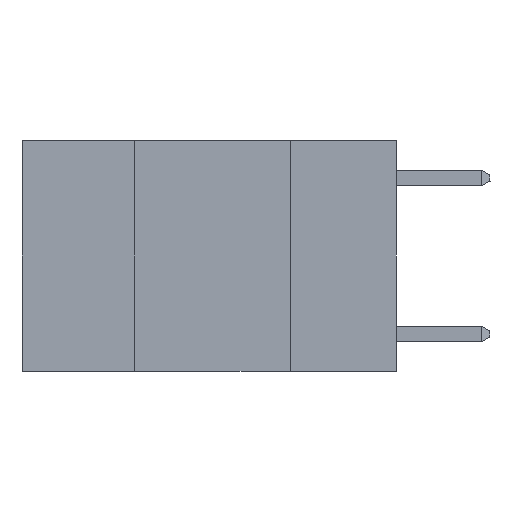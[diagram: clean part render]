
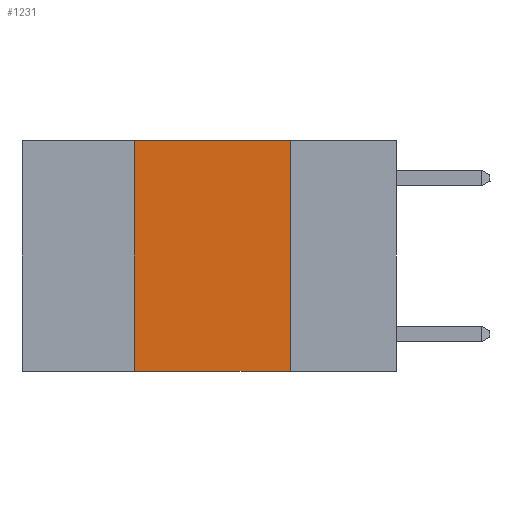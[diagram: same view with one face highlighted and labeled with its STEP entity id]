
A CAD part, left-side view. The second image highlights one B-rep face of the part: STEP entity #1231.
In plain terms, the highlighted planar face has unit normal (-1, 0, 0).
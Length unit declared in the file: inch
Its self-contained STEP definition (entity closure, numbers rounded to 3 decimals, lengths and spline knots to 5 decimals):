
#757 = VECTOR ( 'NONE', #13099, 39.37008 ) ;
#1231 = ADVANCED_FACE ( 'NONE', ( #10437 ), #6418, .F. ) ;
#1411 = CARTESIAN_POINT ( 'NONE',  ( 0., 0.42, -0.37 ) ) ;
#2213 = EDGE_LOOP ( 'NONE', ( #12936, #3602, #9291, #8580 ) ) ;
#2534 = CARTESIAN_POINT ( 'NONE',  ( 0., 0.17, 0. ) ) ;
#2697 = LINE ( 'NONE', #8985, #3651 ) ;
#3078 = DIRECTION ( 'NONE',  ( 1., 0., 0. ) ) ;
#3287 = VERTEX_POINT ( 'NONE', #4025 ) ;
#3602 = ORIENTED_EDGE ( 'NONE', *, *, #9061, .F. ) ;
#3651 = VECTOR ( 'NONE', #9928, 39.37008 ) ;
#4025 = CARTESIAN_POINT ( 'NONE',  ( 0., 0.17, -0.37 ) ) ;
#4538 = VECTOR ( 'NONE', #5242, 39.37008 ) ;
#4675 = CARTESIAN_POINT ( 'NONE',  ( 0., 0.42, 0. ) ) ;
#4904 = EDGE_CURVE ( 'NONE', #11406, #3287, #12012, .T. ) ;
#5172 = VECTOR ( 'NONE', #10143, 39.37008 ) ;
#5242 = DIRECTION ( 'NONE',  ( 0., 0., 1. ) ) ;
#5466 = CARTESIAN_POINT ( 'NONE',  ( 0., 0.6, 0. ) ) ;
#6418 = PLANE ( 'NONE',  #7276 ) ;
#7038 = CARTESIAN_POINT ( 'NONE',  ( 0., 0.6, -0.37 ) ) ;
#7265 = DIRECTION ( 'NONE',  ( 0., 0., -1. ) ) ;
#7276 = AXIS2_PLACEMENT_3D ( 'NONE', #5466, #3078, #7265 ) ;
#7347 = EDGE_CURVE ( 'NONE', #10371, #3287, #7853, .T. ) ;
#7853 = LINE ( 'NONE', #7038, #5172 ) ;
#8580 = ORIENTED_EDGE ( 'NONE', *, *, #7347, .T. ) ;
#8985 = CARTESIAN_POINT ( 'NONE',  ( 0., 0.6, 0. ) ) ;
#9061 = EDGE_CURVE ( 'NONE', #12793, #11406, #2697, .T. ) ;
#9291 = ORIENTED_EDGE ( 'NONE', *, *, #10584, .F. ) ;
#9928 = DIRECTION ( 'NONE',  ( 0., -1., 0. ) ) ;
#9943 = CARTESIAN_POINT ( 'NONE',  ( 0., 0.17, 0. ) ) ;
#10143 = DIRECTION ( 'NONE',  ( 0., -1., 0. ) ) ;
#10267 = LINE ( 'NONE', #10484, #4538 ) ;
#10371 = VERTEX_POINT ( 'NONE', #1411 ) ;
#10437 = FACE_OUTER_BOUND ( 'NONE', #2213, .T. ) ;
#10484 = CARTESIAN_POINT ( 'NONE',  ( 0., 0.42, 0. ) ) ;
#10584 = EDGE_CURVE ( 'NONE', #10371, #12793, #10267, .T. ) ;
#11406 = VERTEX_POINT ( 'NONE', #2534 ) ;
#12012 = LINE ( 'NONE', #9943, #757 ) ;
#12793 = VERTEX_POINT ( 'NONE', #4675 ) ;
#12936 = ORIENTED_EDGE ( 'NONE', *, *, #4904, .F. ) ;
#13099 = DIRECTION ( 'NONE',  ( 0., 0., -1. ) ) ;
